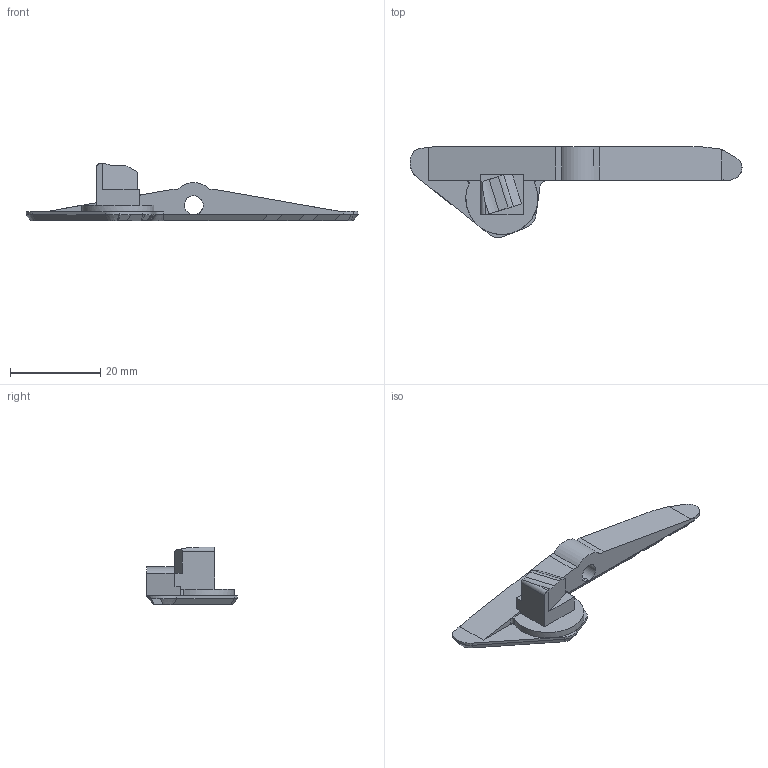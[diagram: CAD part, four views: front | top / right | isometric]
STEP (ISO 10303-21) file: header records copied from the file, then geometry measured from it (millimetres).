
FILE_DESCRIPTION(/* description */ (''),/* implementation_level */ '2;1');
FILE_NAME(/* name */ 'Magazine Catch Bar.step',/* time_stamp */ '2022-05-12T09:40:47-06:00',/* author */ (''),/* organization */ (''),/* preprocessor_version */ 'ST-DEVELOPER v18.1',/* originating_system */ 'Autodesk Translation Framework v10.10.0.1391',/* authorisation */ '');
FILE_SCHEMA (('AUTOMOTIVE_DESIGN { 1 0 10303 214 3 1 1 }'));
Length unit declared in the file: millimetre
Products named in the file (1): Magazine Catch Bar
Bounding box: 73.72 x 20.18 x 12.88 mm (x, y, z)
Volume: 3265 mm3; surface area: 2702.4 mm2
Topology: 1 solids, 3 shells, 134 faces, 335 edges, 205 vertices
Faces by surface type: plane 83, cylinder 24, bspline 14, cone 12, torus 1
Full cylindrical faces by diameter (mm): 4.2 x1
Entity records: 4362 total; most frequent: CARTESIAN_POINT 1207, ORIENTED_EDGE 670, DIRECTION 613, EDGE_CURVE 335, LINE 223, VECTOR 223, VERTEX_POINT 205, AXIS2_PLACEMENT_3D 195
